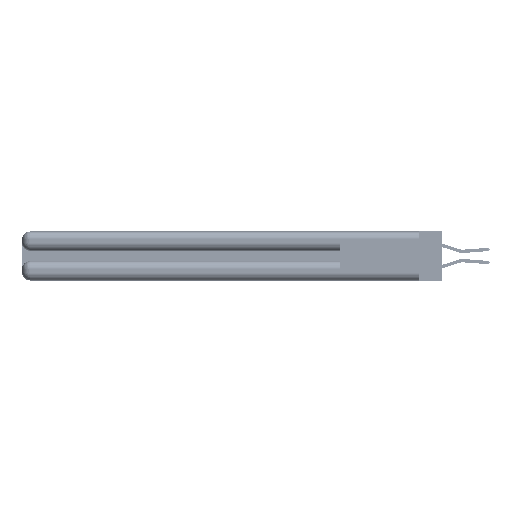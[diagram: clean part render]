
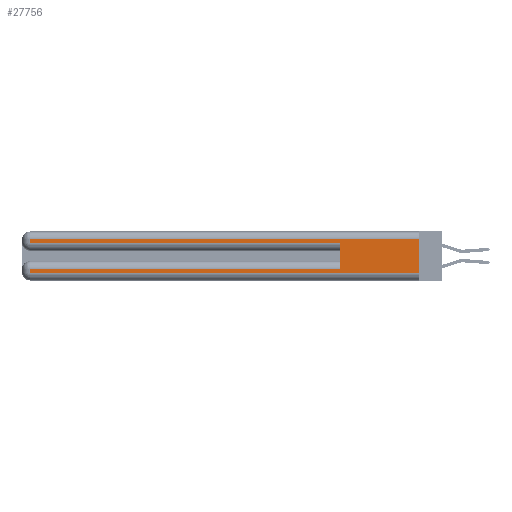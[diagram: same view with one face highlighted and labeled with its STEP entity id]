
A CAD part, left-side view. The second image highlights one B-rep face of the part: STEP entity #27756.
In plain terms, the highlighted planar face has unit normal (-1, 0, 0).
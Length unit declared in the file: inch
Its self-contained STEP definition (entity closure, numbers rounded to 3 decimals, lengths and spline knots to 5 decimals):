
#2369 = PLANE ( 'NONE',  #11196 ) ;
#3507 = EDGE_CURVE ( 'NONE', #37689, #25028, #9342, .T. ) ;
#4100 = DIRECTION ( 'NONE',  ( 1., 0., 0. ) ) ;
#6049 = CARTESIAN_POINT ( 'NONE',  ( 0., 0., 0.06 ) ) ;
#7031 = EDGE_CURVE ( 'NONE', #37689, #36395, #25160, .T. ) ;
#7367 = ORIENTED_EDGE ( 'NONE', *, *, #7031, .T. ) ;
#8231 = CARTESIAN_POINT ( 'NONE',  ( 0., 2.94, 0.285 ) ) ;
#9221 = LINE ( 'NONE', #51801, #51629 ) ;
#9342 = LINE ( 'NONE', #50389, #55797 ) ;
#11196 = AXIS2_PLACEMENT_3D ( 'NONE', #30261, #4100, #55647 ) ;
#12895 = CARTESIAN_POINT ( 'NONE',  ( 0., 0., 0.31 ) ) ;
#12963 = EDGE_CURVE ( 'NONE', #36395, #29362, #45120, .T. ) ;
#14038 = VERTEX_POINT ( 'NONE', #41545 ) ;
#14219 = ORIENTED_EDGE ( 'NONE', *, *, #33817, .F. ) ;
#14623 = VECTOR ( 'NONE', #30064, 39.37008 ) ;
#14704 = CARTESIAN_POINT ( 'NONE',  ( 0., 2.94, 0.31 ) ) ;
#15496 = VECTOR ( 'NONE', #52462, 39.37008 ) ;
#16064 = EDGE_CURVE ( 'NONE', #29362, #49965, #25547, .T. ) ;
#16927 = ORIENTED_EDGE ( 'NONE', *, *, #45065, .T. ) ;
#17460 = ORIENTED_EDGE ( 'NONE', *, *, #16064, .T. ) ;
#18555 = ORIENTED_EDGE ( 'NONE', *, *, #12963, .T. ) ;
#18684 = CARTESIAN_POINT ( 'NONE',  ( 0., 0.6, 0.145 ) ) ;
#18990 = VERTEX_POINT ( 'NONE', #26505 ) ;
#19958 = VECTOR ( 'NONE', #21779, 39.37008 ) ;
#20638 = LINE ( 'NONE', #52957, #19958 ) ;
#21214 = LINE ( 'NONE', #18684, #35538 ) ;
#21779 = DIRECTION ( 'NONE',  ( 0., 0., -1. ) ) ;
#22978 = CARTESIAN_POINT ( 'NONE',  ( 0., 0.6, 0.285 ) ) ;
#23892 = CARTESIAN_POINT ( 'NONE',  ( 0., 0., 0.31 ) ) ;
#25028 = VERTEX_POINT ( 'NONE', #6049 ) ;
#25160 = LINE ( 'NONE', #12895, #31320 ) ;
#25406 = CARTESIAN_POINT ( 'NONE',  ( 0., 2.94, 0.06 ) ) ;
#25547 = LINE ( 'NONE', #56228, #14623 ) ;
#26505 = CARTESIAN_POINT ( 'NONE',  ( 0., 0.6, 0.085 ) ) ;
#27756 = ADVANCED_FACE ( 'NONE', ( #49837 ), #2369, .F. ) ;
#29362 = VERTEX_POINT ( 'NONE', #8231 ) ;
#30064 = DIRECTION ( 'NONE',  ( 0., -1., 0. ) ) ;
#30261 = CARTESIAN_POINT ( 'NONE',  ( 0., 0., 0.37 ) ) ;
#30310 = CARTESIAN_POINT ( 'NONE',  ( 0., 0., 0.085 ) ) ;
#30522 = ORIENTED_EDGE ( 'NONE', *, *, #37983, .T. ) ;
#30630 = DIRECTION ( 'NONE',  ( 0., 1., 0. ) ) ;
#31320 = VECTOR ( 'NONE', #30630, 39.37008 ) ;
#33144 = ORIENTED_EDGE ( 'NONE', *, *, #3507, .F. ) ;
#33481 = VECTOR ( 'NONE', #36398, 39.37008 ) ;
#33817 = EDGE_CURVE ( 'NONE', #18990, #49965, #21214, .T. ) ;
#34498 = EDGE_LOOP ( 'NONE', ( #33144, #7367, #18555, #17460, #14219, #43841, #16927, #30522 ) ) ;
#35538 = VECTOR ( 'NONE', #45597, 39.37008 ) ;
#36395 = VERTEX_POINT ( 'NONE', #14704 ) ;
#36398 = DIRECTION ( 'NONE',  ( 0., 0., -1. ) ) ;
#37689 = VERTEX_POINT ( 'NONE', #23892 ) ;
#37983 = EDGE_CURVE ( 'NONE', #51235, #25028, #9221, .T. ) ;
#41545 = CARTESIAN_POINT ( 'NONE',  ( 0., 2.94, 0.085 ) ) ;
#43841 = ORIENTED_EDGE ( 'NONE', *, *, #55403, .T. ) ;
#45065 = EDGE_CURVE ( 'NONE', #14038, #51235, #20638, .T. ) ;
#45120 = LINE ( 'NONE', #54751, #33481 ) ;
#45597 = DIRECTION ( 'NONE',  ( 0., 0., 1. ) ) ;
#46735 = DIRECTION ( 'NONE',  ( 0., 0., -1. ) ) ;
#46974 = LINE ( 'NONE', #30310, #15496 ) ;
#49837 = FACE_OUTER_BOUND ( 'NONE', #34498, .T. ) ;
#49965 = VERTEX_POINT ( 'NONE', #22978 ) ;
#50389 = CARTESIAN_POINT ( 'NONE',  ( 0., 0., 0.37 ) ) ;
#51235 = VERTEX_POINT ( 'NONE', #25406 ) ;
#51629 = VECTOR ( 'NONE', #56372, 39.37008 ) ;
#51801 = CARTESIAN_POINT ( 'NONE',  ( 0., 0., 0.06 ) ) ;
#52462 = DIRECTION ( 'NONE',  ( 0., 1., 0. ) ) ;
#52957 = CARTESIAN_POINT ( 'NONE',  ( 0., 2.94, 0.37 ) ) ;
#54751 = CARTESIAN_POINT ( 'NONE',  ( 0., 2.94, 0.37 ) ) ;
#55403 = EDGE_CURVE ( 'NONE', #18990, #14038, #46974, .T. ) ;
#55647 = DIRECTION ( 'NONE',  ( 0., 0., -1. ) ) ;
#55797 = VECTOR ( 'NONE', #46735, 39.37008 ) ;
#56228 = CARTESIAN_POINT ( 'NONE',  ( 0., 0., 0.285 ) ) ;
#56372 = DIRECTION ( 'NONE',  ( 0., -1., 0. ) ) ;
